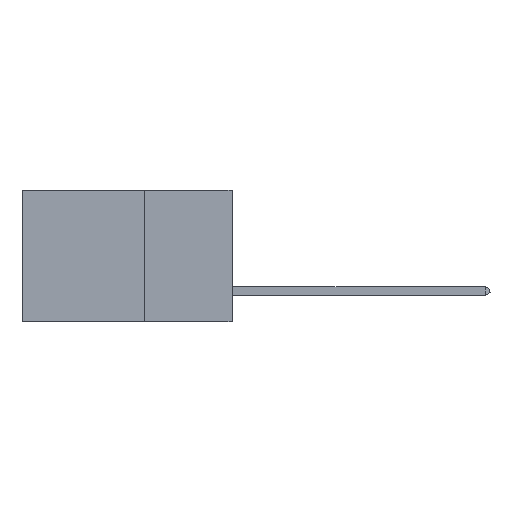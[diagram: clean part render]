
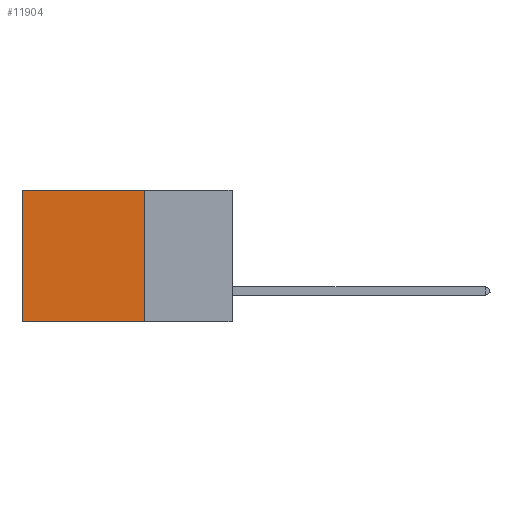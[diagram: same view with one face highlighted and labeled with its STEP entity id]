
A CAD part, left-side view. The second image highlights one B-rep face of the part: STEP entity #11904.
In plain terms, the highlighted planar face has unit normal (-1, 0, 0).
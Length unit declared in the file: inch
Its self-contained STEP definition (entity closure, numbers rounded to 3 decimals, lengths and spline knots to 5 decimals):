
#137 = FACE_OUTER_BOUND ( 'NONE', #8824, .T. ) ;
#872 = EDGE_CURVE ( 'NONE', #2317, #2331, #13799, .T. ) ;
#1992 = DIRECTION ( 'NONE',  ( 0., 0., -1. ) ) ;
#2317 = VERTEX_POINT ( 'NONE', #10737 ) ;
#2331 = VERTEX_POINT ( 'NONE', #8592 ) ;
#2926 = CARTESIAN_POINT ( 'NONE',  ( 0.2875, 0.6, -0.375 ) ) ;
#3216 = DIRECTION ( 'NONE',  ( 1., 0., 0. ) ) ;
#3224 = CARTESIAN_POINT ( 'NONE',  ( 0.2875, 0.6, -0.375 ) ) ;
#3269 = VECTOR ( 'NONE', #10815, 39.37008 ) ;
#3448 = LINE ( 'NONE', #8692, #8268 ) ;
#4302 = DIRECTION ( 'NONE',  ( 0., 0., -1. ) ) ;
#4590 = EDGE_CURVE ( 'NONE', #7219, #8375, #7308, .T. ) ;
#4640 = VECTOR ( 'NONE', #1992, 39.37008 ) ;
#4717 = EDGE_CURVE ( 'NONE', #2331, #8375, #12757, .T. ) ;
#4916 = DIRECTION ( 'NONE',  ( 0., 1., 0. ) ) ;
#5024 = ORIENTED_EDGE ( 'NONE', *, *, #11439, .F. ) ;
#5098 = AXIS2_PLACEMENT_3D ( 'NONE', #5448, #3216, #4302 ) ;
#5448 = CARTESIAN_POINT ( 'NONE',  ( 0.2875, 0.25, -0.375 ) ) ;
#5593 = PLANE ( 'NONE',  #5098 ) ;
#5921 = CARTESIAN_POINT ( 'NONE',  ( 0.2875, 0.25, 0. ) ) ;
#6438 = VECTOR ( 'NONE', #4916, 39.37008 ) ;
#7219 = VERTEX_POINT ( 'NONE', #11776 ) ;
#7308 = LINE ( 'NONE', #12690, #3269 ) ;
#8268 = VECTOR ( 'NONE', #13071, 39.37008 ) ;
#8375 = VERTEX_POINT ( 'NONE', #3224 ) ;
#8592 = CARTESIAN_POINT ( 'NONE',  ( 0.2875, 0.6, 0. ) ) ;
#8692 = CARTESIAN_POINT ( 'NONE',  ( 0.2875, 0.25, -0.375 ) ) ;
#8824 = EDGE_LOOP ( 'NONE', ( #9827, #9323, #5024, #12097 ) ) ;
#9323 = ORIENTED_EDGE ( 'NONE', *, *, #4590, .F. ) ;
#9827 = ORIENTED_EDGE ( 'NONE', *, *, #4717, .T. ) ;
#10737 = CARTESIAN_POINT ( 'NONE',  ( 0.2875, 0.25, 0. ) ) ;
#10815 = DIRECTION ( 'NONE',  ( 0., 1., 0. ) ) ;
#11439 = EDGE_CURVE ( 'NONE', #2317, #7219, #3448, .T. ) ;
#11776 = CARTESIAN_POINT ( 'NONE',  ( 0.2875, 0.25, -0.375 ) ) ;
#11904 = ADVANCED_FACE ( 'NONE', ( #137 ), #5593, .F. ) ;
#12097 = ORIENTED_EDGE ( 'NONE', *, *, #872, .T. ) ;
#12690 = CARTESIAN_POINT ( 'NONE',  ( 0.2875, 0.25, -0.375 ) ) ;
#12757 = LINE ( 'NONE', #2926, #4640 ) ;
#13071 = DIRECTION ( 'NONE',  ( 0., 0., -1. ) ) ;
#13799 = LINE ( 'NONE', #5921, #6438 ) ;
